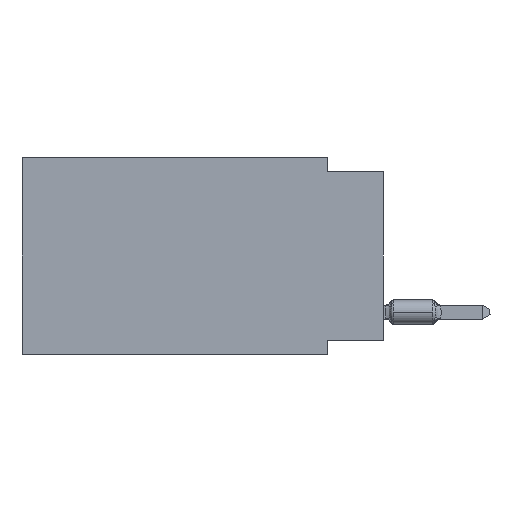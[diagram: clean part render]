
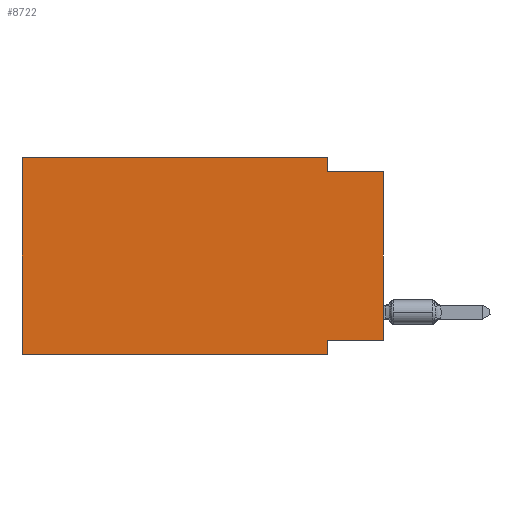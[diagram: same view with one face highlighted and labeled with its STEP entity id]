
A CAD part, left-side view. The second image highlights one B-rep face of the part: STEP entity #8722.
In plain terms, the highlighted planar face has unit normal (-1, 0, 0).
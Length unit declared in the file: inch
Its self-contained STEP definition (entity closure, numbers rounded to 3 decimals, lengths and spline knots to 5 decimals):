
#167 = EDGE_CURVE ( 'NONE', #9064, #19709, #14410, .T. ) ;
#614 = PLANE ( 'NONE',  #22598 ) ;
#815 = EDGE_CURVE ( 'NONE', #15641, #19709, #9448, .T. ) ;
#860 = CARTESIAN_POINT ( 'NONE',  ( 0., 0.1, 0. ) ) ;
#1588 = DIRECTION ( 'NONE',  ( 0., 1., 0. ) ) ;
#1617 = VECTOR ( 'NONE', #6434, 39.37008 ) ;
#1694 = LINE ( 'NONE', #11050, #20255 ) ;
#1754 = EDGE_CURVE ( 'NONE', #19689, #10402, #17704, .T. ) ;
#2171 = DIRECTION ( 'NONE',  ( 0., 0., -1. ) ) ;
#2420 = CARTESIAN_POINT ( 'NONE',  ( 0., 0.645, 0. ) ) ;
#2463 = CARTESIAN_POINT ( 'NONE',  ( 0., 0.645, 0. ) ) ;
#2762 = ORIENTED_EDGE ( 'NONE', *, *, #815, .F. ) ;
#2922 = ORIENTED_EDGE ( 'NONE', *, *, #8887, .T. ) ;
#3105 = ORIENTED_EDGE ( 'NONE', *, *, #1754, .F. ) ;
#3558 = CARTESIAN_POINT ( 'NONE',  ( 0., 0.645, 0. ) ) ;
#3620 = CARTESIAN_POINT ( 'NONE',  ( 0., 0.645, 0. ) ) ;
#3637 = ORIENTED_EDGE ( 'NONE', *, *, #12432, .F. ) ;
#4420 = VECTOR ( 'NONE', #10459, 39.37008 ) ;
#5790 = CARTESIAN_POINT ( 'NONE',  ( 0., 0.1, 0. ) ) ;
#6434 = DIRECTION ( 'NONE',  ( 0., -1., 0. ) ) ;
#6555 = CARTESIAN_POINT ( 'NONE',  ( 0., 0.645, -0.35 ) ) ;
#7366 = VECTOR ( 'NONE', #17409, 39.37008 ) ;
#7713 = LINE ( 'NONE', #2420, #7366 ) ;
#7882 = DIRECTION ( 'NONE',  ( 1., 0., 0. ) ) ;
#8343 = VECTOR ( 'NONE', #1588, 39.37008 ) ;
#8722 = ADVANCED_FACE ( 'NONE', ( #19292 ), #614, .F. ) ;
#8887 = EDGE_CURVE ( 'NONE', #21491, #9219, #1694, .T. ) ;
#9064 = VERTEX_POINT ( 'NONE', #15323 ) ;
#9074 = VECTOR ( 'NONE', #20747, 39.37008 ) ;
#9219 = VERTEX_POINT ( 'NONE', #12495 ) ;
#9448 = LINE ( 'NONE', #17050, #9580 ) ;
#9580 = VECTOR ( 'NONE', #2171, 39.37008 ) ;
#10402 = VERTEX_POINT ( 'NONE', #15057 ) ;
#10459 = DIRECTION ( 'NONE',  ( 0., 0., -1. ) ) ;
#11050 = CARTESIAN_POINT ( 'NONE',  ( 0., 0., 0. ) ) ;
#11411 = CARTESIAN_POINT ( 'NONE',  ( 0., 0., -0.025 ) ) ;
#11965 = ORIENTED_EDGE ( 'NONE', *, *, #12317, .F. ) ;
#12053 = ORIENTED_EDGE ( 'NONE', *, *, #167, .T. ) ;
#12317 = EDGE_CURVE ( 'NONE', #21491, #15641, #21628, .T. ) ;
#12432 = EDGE_CURVE ( 'NONE', #10402, #9219, #22354, .T. ) ;
#12495 = CARTESIAN_POINT ( 'NONE',  ( 0., 0., -0.025 ) ) ;
#12567 = VERTEX_POINT ( 'NONE', #3620 ) ;
#13116 = DIRECTION ( 'NONE',  ( 0., 0., 1. ) ) ;
#13506 = DIRECTION ( 'NONE',  ( 0., 0., -1. ) ) ;
#14410 = LINE ( 'NONE', #6555, #1617 ) ;
#14462 = CARTESIAN_POINT ( 'NONE',  ( 0., 0., -0.325 ) ) ;
#15057 = CARTESIAN_POINT ( 'NONE',  ( 0., 0.1, -0.025 ) ) ;
#15287 = ORIENTED_EDGE ( 'NONE', *, *, #23798, .F. ) ;
#15323 = CARTESIAN_POINT ( 'NONE',  ( 0., 0.645, -0.35 ) ) ;
#15406 = EDGE_LOOP ( 'NONE', ( #2922, #3637, #3105, #15287, #22380, #12053, #2762, #11965 ) ) ;
#15641 = VERTEX_POINT ( 'NONE', #22832 ) ;
#15899 = VECTOR ( 'NONE', #21744, 39.37008 ) ;
#17050 = CARTESIAN_POINT ( 'NONE',  ( 0., 0.1, -0.35 ) ) ;
#17243 = EDGE_CURVE ( 'NONE', #9064, #12567, #7713, .T. ) ;
#17409 = DIRECTION ( 'NONE',  ( 0., 0., 1. ) ) ;
#17704 = LINE ( 'NONE', #860, #4420 ) ;
#18070 = LINE ( 'NONE', #3558, #15899 ) ;
#18429 = CARTESIAN_POINT ( 'NONE',  ( 0., 0., -0.325 ) ) ;
#19292 = FACE_OUTER_BOUND ( 'NONE', #15406, .T. ) ;
#19402 = CARTESIAN_POINT ( 'NONE',  ( 0., 0.1, -0.35 ) ) ;
#19689 = VERTEX_POINT ( 'NONE', #5790 ) ;
#19709 = VERTEX_POINT ( 'NONE', #19402 ) ;
#20255 = VECTOR ( 'NONE', #13116, 39.37008 ) ;
#20747 = DIRECTION ( 'NONE',  ( 0., -1., 0. ) ) ;
#21491 = VERTEX_POINT ( 'NONE', #14462 ) ;
#21628 = LINE ( 'NONE', #18429, #8343 ) ;
#21744 = DIRECTION ( 'NONE',  ( 0., -1., 0. ) ) ;
#22354 = LINE ( 'NONE', #11411, #9074 ) ;
#22380 = ORIENTED_EDGE ( 'NONE', *, *, #17243, .F. ) ;
#22598 = AXIS2_PLACEMENT_3D ( 'NONE', #2463, #7882, #13506 ) ;
#22832 = CARTESIAN_POINT ( 'NONE',  ( 0., 0.1, -0.325 ) ) ;
#23798 = EDGE_CURVE ( 'NONE', #12567, #19689, #18070, .T. ) ;
